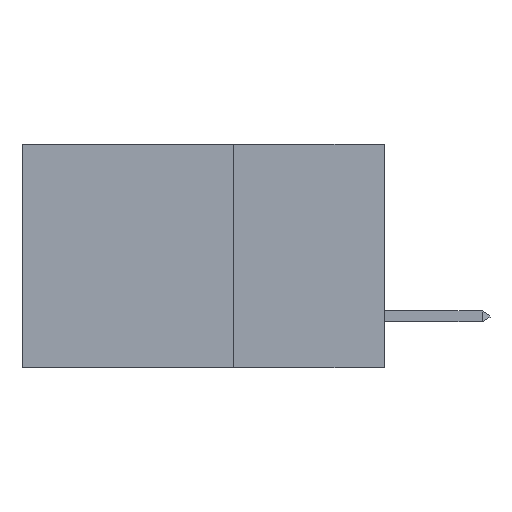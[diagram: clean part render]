
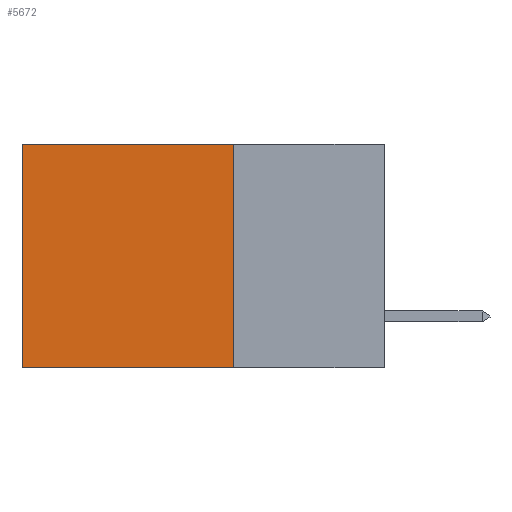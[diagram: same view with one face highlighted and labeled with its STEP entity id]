
A CAD part, left-side view. The second image highlights one B-rep face of the part: STEP entity #5672.
In plain terms, the highlighted planar face has unit normal (-1, 0, 0).
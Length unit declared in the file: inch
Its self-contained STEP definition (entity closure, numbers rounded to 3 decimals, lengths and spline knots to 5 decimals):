
#527 = EDGE_CURVE ( 'NONE', #14226, #9133, #8746, .T. ) ;
#582 = VERTEX_POINT ( 'NONE', #2089 ) ;
#642 = DIRECTION ( 'NONE',  ( 0., 1., 0. ) ) ;
#678 = DIRECTION ( 'NONE',  ( 1., 0., 0. ) ) ;
#774 = CARTESIAN_POINT ( 'NONE',  ( 0.2875, 0.6, 0. ) ) ;
#1843 = EDGE_CURVE ( 'NONE', #9133, #582, #12572, .T. ) ;
#1874 = ORIENTED_EDGE ( 'NONE', *, *, #1843, .F. ) ;
#2089 = CARTESIAN_POINT ( 'NONE',  ( 0.2875, 0.6, -0.37 ) ) ;
#2285 = LINE ( 'NONE', #8838, #10826 ) ;
#2752 = VECTOR ( 'NONE', #7438, 39.37008 ) ;
#3396 = ORIENTED_EDGE ( 'NONE', *, *, #527, .F. ) ;
#4042 = CARTESIAN_POINT ( 'NONE',  ( 0.2875, 0.6, 0. ) ) ;
#4709 = EDGE_LOOP ( 'NONE', ( #6870, #1874, #3396, #4805 ) ) ;
#4805 = ORIENTED_EDGE ( 'NONE', *, *, #11056, .T. ) ;
#5647 = DIRECTION ( 'NONE',  ( 0., 0., -1. ) ) ;
#5672 = ADVANCED_FACE ( 'NONE', ( #8963 ), #11907, .F. ) ;
#5958 = VECTOR ( 'NONE', #5647, 39.37008 ) ;
#6678 = VECTOR ( 'NONE', #11959, 39.37008 ) ;
#6870 = ORIENTED_EDGE ( 'NONE', *, *, #13737, .T. ) ;
#7438 = DIRECTION ( 'NONE',  ( 0., 0., -1. ) ) ;
#7976 = VERTEX_POINT ( 'NONE', #4042 ) ;
#8746 = LINE ( 'NONE', #11735, #2752 ) ;
#8838 = CARTESIAN_POINT ( 'NONE',  ( 0.2875, 0.25, 0. ) ) ;
#8863 = DIRECTION ( 'NONE',  ( 0., 0., -1. ) ) ;
#8963 = FACE_OUTER_BOUND ( 'NONE', #4709, .T. ) ;
#9009 = AXIS2_PLACEMENT_3D ( 'NONE', #13906, #678, #8863 ) ;
#9133 = VERTEX_POINT ( 'NONE', #14216 ) ;
#10826 = VECTOR ( 'NONE', #642, 39.37008 ) ;
#11056 = EDGE_CURVE ( 'NONE', #14226, #7976, #2285, .T. ) ;
#11710 = CARTESIAN_POINT ( 'NONE',  ( 0.2875, 0.25, 0. ) ) ;
#11735 = CARTESIAN_POINT ( 'NONE',  ( 0.2875, 0.25, 0. ) ) ;
#11854 = CARTESIAN_POINT ( 'NONE',  ( 0.2875, 0.25, -0.37 ) ) ;
#11907 = PLANE ( 'NONE',  #9009 ) ;
#11959 = DIRECTION ( 'NONE',  ( 0., 1., 0. ) ) ;
#12572 = LINE ( 'NONE', #11854, #6678 ) ;
#13737 = EDGE_CURVE ( 'NONE', #7976, #582, #14306, .T. ) ;
#13906 = CARTESIAN_POINT ( 'NONE',  ( 0.2875, 0.25, 0. ) ) ;
#14216 = CARTESIAN_POINT ( 'NONE',  ( 0.2875, 0.25, -0.37 ) ) ;
#14226 = VERTEX_POINT ( 'NONE', #11710 ) ;
#14306 = LINE ( 'NONE', #774, #5958 ) ;
